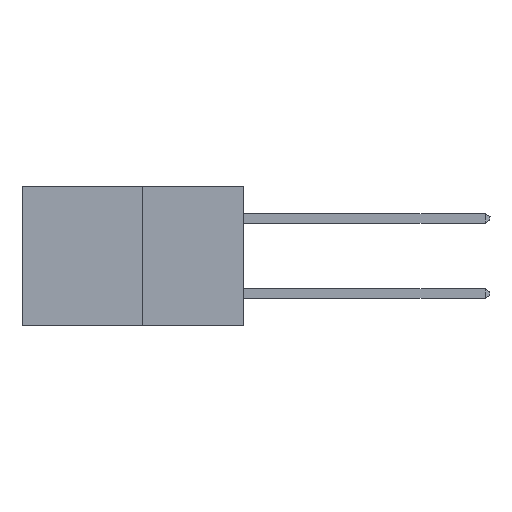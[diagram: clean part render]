
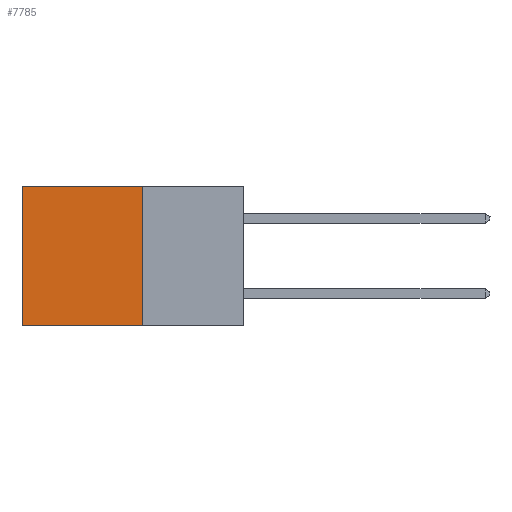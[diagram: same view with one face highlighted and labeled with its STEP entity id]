
A CAD part, left-side view. The second image highlights one B-rep face of the part: STEP entity #7785.
In plain terms, the highlighted planar face has unit normal (-1, 0, 0).
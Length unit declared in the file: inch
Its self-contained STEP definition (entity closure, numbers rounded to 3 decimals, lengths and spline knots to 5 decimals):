
#373 = FACE_OUTER_BOUND ( 'NONE', #5325, .T. ) ;
#522 = CARTESIAN_POINT ( 'NONE',  ( 0.277, 0.27, 0. ) ) ;
#561 = DIRECTION ( 'NONE',  ( 0., 0., -1. ) ) ;
#667 = ORIENTED_EDGE ( 'NONE', *, *, #10005, .F. ) ;
#1517 = ORIENTED_EDGE ( 'NONE', *, *, #4153, .T. ) ;
#1637 = CARTESIAN_POINT ( 'NONE',  ( 0.277, 0.27, -0.37 ) ) ;
#1955 = VECTOR ( 'NONE', #9628, 39.37008 ) ;
#2773 = ORIENTED_EDGE ( 'NONE', *, *, #4507, .T. ) ;
#2783 = VERTEX_POINT ( 'NONE', #3611 ) ;
#3551 = CARTESIAN_POINT ( 'NONE',  ( 0.277, 0.59, -0.37 ) ) ;
#3611 = CARTESIAN_POINT ( 'NONE',  ( 0.277, 0.27, -0.37 ) ) ;
#3654 = LINE ( 'NONE', #10304, #8003 ) ;
#4153 = EDGE_CURVE ( 'NONE', #7606, #7163, #10343, .T. ) ;
#4222 = ORIENTED_EDGE ( 'NONE', *, *, #7611, .F. ) ;
#4507 = EDGE_CURVE ( 'NONE', #7163, #4643, #9501, .T. ) ;
#4643 = VERTEX_POINT ( 'NONE', #9427 ) ;
#4856 = AXIS2_PLACEMENT_3D ( 'NONE', #1637, #10611, #5830 ) ;
#5001 = PLANE ( 'NONE',  #4856 ) ;
#5048 = CARTESIAN_POINT ( 'NONE',  ( 0.277, 0.59, 0. ) ) ;
#5325 = EDGE_LOOP ( 'NONE', ( #2773, #667, #4222, #1517 ) ) ;
#5492 = DIRECTION ( 'NONE',  ( 0., 1., 0. ) ) ;
#5576 = CARTESIAN_POINT ( 'NONE',  ( 0.277, 0.27, -0.37 ) ) ;
#5830 = DIRECTION ( 'NONE',  ( 0., 0., -1. ) ) ;
#6145 = VECTOR ( 'NONE', #561, 39.37008 ) ;
#7163 = VERTEX_POINT ( 'NONE', #5048 ) ;
#7389 = VECTOR ( 'NONE', #8439, 39.37008 ) ;
#7606 = VERTEX_POINT ( 'NONE', #522 ) ;
#7611 = EDGE_CURVE ( 'NONE', #7606, #2783, #8291, .T. ) ;
#7785 = ADVANCED_FACE ( 'NONE', ( #373 ), #5001, .F. ) ;
#8003 = VECTOR ( 'NONE', #5492, 39.37008 ) ;
#8291 = LINE ( 'NONE', #5576, #6145 ) ;
#8439 = DIRECTION ( 'NONE',  ( 0., 0., -1. ) ) ;
#8832 = CARTESIAN_POINT ( 'NONE',  ( 0.277, 0.27, 0. ) ) ;
#9427 = CARTESIAN_POINT ( 'NONE',  ( 0.277, 0.59, -0.37 ) ) ;
#9501 = LINE ( 'NONE', #3551, #7389 ) ;
#9628 = DIRECTION ( 'NONE',  ( 0., 1., 0. ) ) ;
#10005 = EDGE_CURVE ( 'NONE', #2783, #4643, #3654, .T. ) ;
#10304 = CARTESIAN_POINT ( 'NONE',  ( 0.277, 0.27, -0.37 ) ) ;
#10343 = LINE ( 'NONE', #8832, #1955 ) ;
#10611 = DIRECTION ( 'NONE',  ( 1., 0., 0. ) ) ;
